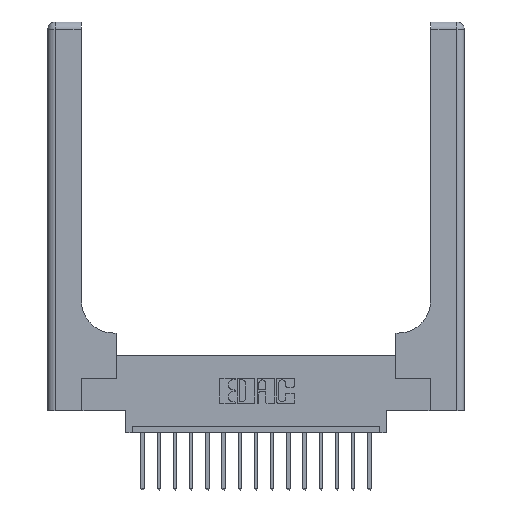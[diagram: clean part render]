
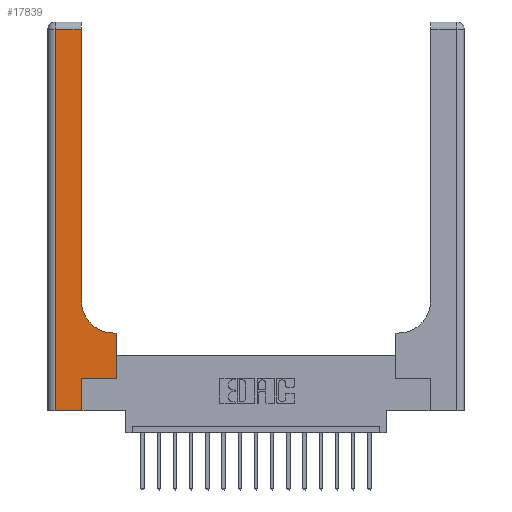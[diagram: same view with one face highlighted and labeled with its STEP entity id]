
A CAD part, top view. The second image highlights one B-rep face of the part: STEP entity #17839.
In plain terms, the highlighted planar face has unit normal (0, 0, 1).
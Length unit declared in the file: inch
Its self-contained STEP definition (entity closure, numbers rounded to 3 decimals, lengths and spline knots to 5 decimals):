
#317 = VERTEX_POINT ( 'NONE', #3705 ) ;
#678 = VECTOR ( 'NONE', #18240, 39.37008 ) ;
#698 = ORIENTED_EDGE ( 'NONE', *, *, #16093, .T. ) ;
#788 = DIRECTION ( 'NONE',  ( 0., 1., 0. ) ) ;
#942 = CARTESIAN_POINT ( 'NONE',  ( 0., 2.94, 0.37 ) ) ;
#1070 = CARTESIAN_POINT ( 'NONE',  ( 0.06, 0., 0.37 ) ) ;
#2169 = LINE ( 'NONE', #5008, #678 ) ;
#2240 = ORIENTED_EDGE ( 'NONE', *, *, #12132, .T. ) ;
#2341 = DIRECTION ( 'NONE',  ( 1., 0., 0. ) ) ;
#3344 = VECTOR ( 'NONE', #788, 39.37008 ) ;
#3409 = CARTESIAN_POINT ( 'NONE',  ( 0.26, 0.85, 0.37 ) ) ;
#3546 = LINE ( 'NONE', #9311, #9861 ) ;
#3594 = VECTOR ( 'NONE', #6728, 39.37008 ) ;
#3705 = CARTESIAN_POINT ( 'NONE',  ( 0.26, 2.94, 0.37 ) ) ;
#4012 = CARTESIAN_POINT ( 'NONE',  ( 0.265, 0.25, 0.37 ) ) ;
#4350 = EDGE_LOOP ( 'NONE', ( #17379, #7956, #698, #11595, #2240, #8885, #16877, #12305, #7087 ) ) ;
#4780 = DIRECTION ( 'NONE',  ( 0., 1., 0. ) ) ;
#5008 = CARTESIAN_POINT ( 'NONE',  ( 0.265, 0.25, 0.37 ) ) ;
#5112 = VECTOR ( 'NONE', #5702, 39.37008 ) ;
#5547 = EDGE_CURVE ( 'NONE', #12941, #317, #3546, .T. ) ;
#5686 = FACE_OUTER_BOUND ( 'NONE', #4350, .T. ) ;
#5702 = DIRECTION ( 'NONE',  ( 0., -1., 0. ) ) ;
#5829 = VERTEX_POINT ( 'NONE', #10047 ) ;
#5835 = CIRCLE ( 'NONE', #16408, 0.25 ) ;
#6242 = CARTESIAN_POINT ( 'NONE',  ( 0.528, 0.25, 0.37 ) ) ;
#6465 = CARTESIAN_POINT ( 'NONE',  ( 0.528, 0.25, 0.37 ) ) ;
#6728 = DIRECTION ( 'NONE',  ( -1., 0., 0. ) ) ;
#7087 = ORIENTED_EDGE ( 'NONE', *, *, #12964, .T. ) ;
#7268 = VERTEX_POINT ( 'NONE', #16212 ) ;
#7611 = LINE ( 'NONE', #7698, #16080 ) ;
#7698 = CARTESIAN_POINT ( 'NONE',  ( 0.265, 0., 0.37 ) ) ;
#7956 = ORIENTED_EDGE ( 'NONE', *, *, #14234, .T. ) ;
#7969 = LINE ( 'NONE', #12327, #16279 ) ;
#8020 = DIRECTION ( 'NONE',  ( -1., 0., 0. ) ) ;
#8759 = CARTESIAN_POINT ( 'NONE',  ( 0.06, 2.94, 0.37 ) ) ;
#8885 = ORIENTED_EDGE ( 'NONE', *, *, #12933, .T. ) ;
#8960 = EDGE_CURVE ( 'NONE', #7268, #14841, #9111, .T. ) ;
#9111 = LINE ( 'NONE', #14867, #3594 ) ;
#9261 = DIRECTION ( 'NONE',  ( 0., 0., -1. ) ) ;
#9311 = CARTESIAN_POINT ( 'NONE',  ( 0.26, 3., 0.37 ) ) ;
#9445 = LINE ( 'NONE', #942, #15130 ) ;
#9861 = VECTOR ( 'NONE', #13485, 39.37008 ) ;
#10047 = CARTESIAN_POINT ( 'NONE',  ( 0.265, 0., 0.37 ) ) ;
#10926 = EDGE_CURVE ( 'NONE', #16875, #7268, #13661, .T. ) ;
#11053 = VERTEX_POINT ( 'NONE', #1070 ) ;
#11446 = PLANE ( 'NONE',  #15407 ) ;
#11513 = VERTEX_POINT ( 'NONE', #8759 ) ;
#11595 = ORIENTED_EDGE ( 'NONE', *, *, #16071, .T. ) ;
#11628 = DIRECTION ( 'NONE',  ( -1., 0., 0. ) ) ;
#12132 = EDGE_CURVE ( 'NONE', #5829, #16123, #7611, .T. ) ;
#12305 = ORIENTED_EDGE ( 'NONE', *, *, #8960, .T. ) ;
#12327 = CARTESIAN_POINT ( 'NONE',  ( 0., 0., 0.37 ) ) ;
#12933 = EDGE_CURVE ( 'NONE', #16123, #16875, #2169, .T. ) ;
#12941 = VERTEX_POINT ( 'NONE', #3409 ) ;
#12964 = EDGE_CURVE ( 'NONE', #14841, #12941, #5835, .T. ) ;
#13485 = DIRECTION ( 'NONE',  ( 0., 1., 0. ) ) ;
#13661 = LINE ( 'NONE', #6465, #3344 ) ;
#14234 = EDGE_CURVE ( 'NONE', #317, #11513, #9445, .T. ) ;
#14299 = CARTESIAN_POINT ( 'NONE',  ( 0.06, 3., 0.37 ) ) ;
#14373 = DIRECTION ( 'NONE',  ( 0., 0., -1. ) ) ;
#14841 = VERTEX_POINT ( 'NONE', #15153 ) ;
#14867 = CARTESIAN_POINT ( 'NONE',  ( 0.26, 0.6, 0.37 ) ) ;
#15130 = VECTOR ( 'NONE', #8020, 39.37008 ) ;
#15153 = CARTESIAN_POINT ( 'NONE',  ( 0.51, 0.6, 0.37 ) ) ;
#15285 = CARTESIAN_POINT ( 'NONE',  ( 0.51, 0.85, 0.37 ) ) ;
#15407 = AXIS2_PLACEMENT_3D ( 'NONE', #17124, #14373, #11628 ) ;
#15520 = LINE ( 'NONE', #14299, #5112 ) ;
#16071 = EDGE_CURVE ( 'NONE', #11053, #5829, #7969, .T. ) ;
#16080 = VECTOR ( 'NONE', #4780, 39.37008 ) ;
#16093 = EDGE_CURVE ( 'NONE', #11513, #11053, #15520, .T. ) ;
#16123 = VERTEX_POINT ( 'NONE', #4012 ) ;
#16212 = CARTESIAN_POINT ( 'NONE',  ( 0.528, 0.6, 0.37 ) ) ;
#16279 = VECTOR ( 'NONE', #16766, 39.37008 ) ;
#16408 = AXIS2_PLACEMENT_3D ( 'NONE', #15285, #9261, #2341 ) ;
#16766 = DIRECTION ( 'NONE',  ( 1., 0., 0. ) ) ;
#16875 = VERTEX_POINT ( 'NONE', #6242 ) ;
#16877 = ORIENTED_EDGE ( 'NONE', *, *, #10926, .T. ) ;
#17124 = CARTESIAN_POINT ( 'NONE',  ( 0., 3., 0.37 ) ) ;
#17379 = ORIENTED_EDGE ( 'NONE', *, *, #5547, .T. ) ;
#17839 = ADVANCED_FACE ( 'NONE', ( #5686 ), #11446, .F. ) ;
#18240 = DIRECTION ( 'NONE',  ( 1., 0., 0. ) ) ;
